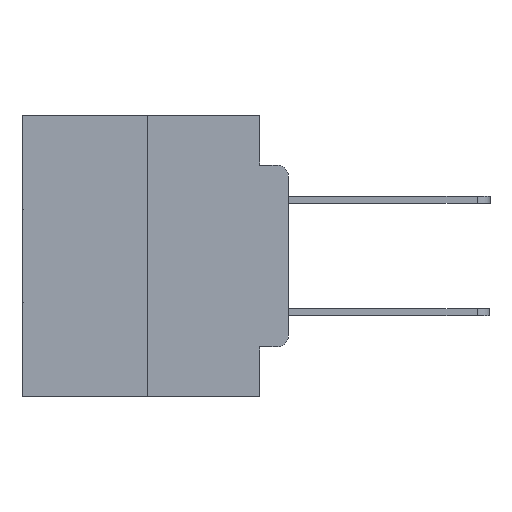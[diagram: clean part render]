
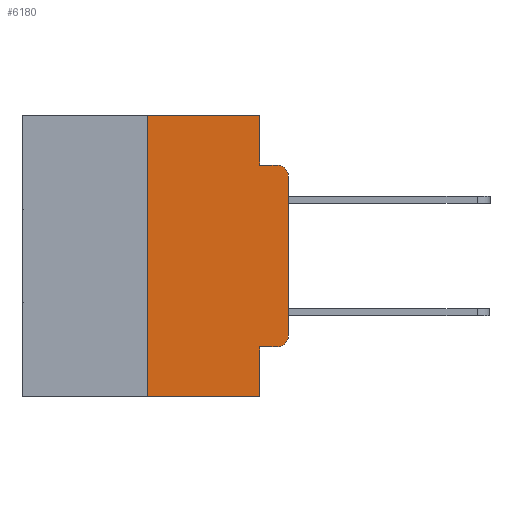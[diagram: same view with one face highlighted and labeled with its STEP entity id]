
A CAD part, left-side view. The second image highlights one B-rep face of the part: STEP entity #6180.
In plain terms, the highlighted planar face has unit normal (-1, 0, 0).
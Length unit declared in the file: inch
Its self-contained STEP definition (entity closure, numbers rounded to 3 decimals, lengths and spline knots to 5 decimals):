
#516 = ORIENTED_EDGE ( 'NONE', *, *, #24378, .F. ) ;
#706 = ORIENTED_EDGE ( 'NONE', *, *, #11833, .T. ) ;
#1183 = CARTESIAN_POINT ( 'NONE',  ( 0., 0.25, 0. ) ) ;
#1330 = ORIENTED_EDGE ( 'NONE', *, *, #25964, .T. ) ;
#2037 = CARTESIAN_POINT ( 'NONE',  ( 0., 0.02, -0.0885 ) ) ;
#2214 = EDGE_CURVE ( 'NONE', #8570, #5010, #18973, .T. ) ;
#3091 = ORIENTED_EDGE ( 'NONE', *, *, #10263, .T. ) ;
#3340 = VECTOR ( 'NONE', #28478, 39.37008 ) ;
#3778 = CARTESIAN_POINT ( 'NONE',  ( 0., 0.051, -0.5 ) ) ;
#3823 = VECTOR ( 'NONE', #24757, 39.37008 ) ;
#4241 = CARTESIAN_POINT ( 'NONE',  ( 0., 0.02, -0.1085 ) ) ;
#4290 = CARTESIAN_POINT ( 'NONE',  ( 0., 0.02, -0.3915 ) ) ;
#5010 = VERTEX_POINT ( 'NONE', #3778 ) ;
#5153 = CARTESIAN_POINT ( 'NONE',  ( 0., 0.473, -0.5 ) ) ;
#5860 = CIRCLE ( 'NONE', #20348, 0.02 ) ;
#6048 = CARTESIAN_POINT ( 'NONE',  ( 0., 0.051, 0. ) ) ;
#6180 = ADVANCED_FACE ( 'NONE', ( #27198 ), #7803, .F. ) ;
#6550 = LINE ( 'NONE', #19392, #23729 ) ;
#6603 = DIRECTION ( 'NONE',  ( 0., 0., -1. ) ) ;
#6663 = DIRECTION ( 'NONE',  ( 0., 0., -1. ) ) ;
#7413 = CIRCLE ( 'NONE', #27313, 0.02 ) ;
#7803 = PLANE ( 'NONE',  #23467 ) ;
#7943 = DIRECTION ( 'NONE',  ( 0., 0., 1. ) ) ;
#7974 = LINE ( 'NONE', #18367, #19681 ) ;
#8391 = VECTOR ( 'NONE', #12218, 39.37008 ) ;
#8570 = VERTEX_POINT ( 'NONE', #23497 ) ;
#8673 = DIRECTION ( 'NONE',  ( 0., -1., 0. ) ) ;
#9435 = ORIENTED_EDGE ( 'NONE', *, *, #27572, .T. ) ;
#9583 = LINE ( 'NONE', #26116, #3340 ) ;
#10008 = EDGE_LOOP ( 'NONE', ( #9435, #1330, #516, #18416, #14697, #24965, #27847, #11110, #706, #3091 ) ) ;
#10093 = DIRECTION ( 'NONE',  ( 0., -1., 0. ) ) ;
#10263 = EDGE_CURVE ( 'NONE', #17204, #16734, #7413, .T. ) ;
#10437 = CARTESIAN_POINT ( 'NONE',  ( 0., 0., -0.3915 ) ) ;
#10920 = CARTESIAN_POINT ( 'NONE',  ( 0., 0.051, -0.4115 ) ) ;
#11110 = ORIENTED_EDGE ( 'NONE', *, *, #14972, .F. ) ;
#11296 = VECTOR ( 'NONE', #7943, 39.37008 ) ;
#11700 = CARTESIAN_POINT ( 'NONE',  ( 0., 0., -0.1085 ) ) ;
#11833 = EDGE_CURVE ( 'NONE', #15055, #17204, #23388, .T. ) ;
#12218 = DIRECTION ( 'NONE',  ( 0., 0., -1. ) ) ;
#12506 = CARTESIAN_POINT ( 'NONE',  ( 0., 0.473, 0. ) ) ;
#14697 = ORIENTED_EDGE ( 'NONE', *, *, #24012, .F. ) ;
#14858 = DIRECTION ( 'NONE',  ( 0., 0., -1. ) ) ;
#14892 = CARTESIAN_POINT ( 'NONE',  ( 0., 0., 0. ) ) ;
#14972 = EDGE_CURVE ( 'NONE', #15055, #5010, #28731, .T. ) ;
#15055 = VERTEX_POINT ( 'NONE', #24970 ) ;
#16073 = CARTESIAN_POINT ( 'NONE',  ( 0., 0.02, -0.4115 ) ) ;
#16244 = VERTEX_POINT ( 'NONE', #18047 ) ;
#16544 = EDGE_CURVE ( 'NONE', #8570, #26471, #9583, .T. ) ;
#16734 = VERTEX_POINT ( 'NONE', #10437 ) ;
#16817 = DIRECTION ( 'NONE',  ( 0., -1., 0. ) ) ;
#17165 = VECTOR ( 'NONE', #8673, 39.37008 ) ;
#17204 = VERTEX_POINT ( 'NONE', #16073 ) ;
#17306 = VERTEX_POINT ( 'NONE', #21075 ) ;
#18047 = CARTESIAN_POINT ( 'NONE',  ( 0., 0.051, -0.0885 ) ) ;
#18113 = EDGE_CURVE ( 'NONE', #17306, #16244, #20836, .T. ) ;
#18267 = VECTOR ( 'NONE', #16817, 39.37008 ) ;
#18367 = CARTESIAN_POINT ( 'NONE',  ( 0., 0.051, -0.0885 ) ) ;
#18416 = ORIENTED_EDGE ( 'NONE', *, *, #18113, .F. ) ;
#18973 = LINE ( 'NONE', #5153, #18267 ) ;
#19392 = CARTESIAN_POINT ( 'NONE',  ( 0., 0.473, 0. ) ) ;
#19681 = VECTOR ( 'NONE', #20729, 39.37008 ) ;
#20348 = AXIS2_PLACEMENT_3D ( 'NONE', #4241, #20626, #6603 ) ;
#20626 = DIRECTION ( 'NONE',  ( -1., 0., 0. ) ) ;
#20674 = DIRECTION ( 'NONE',  ( -1., 0., 0. ) ) ;
#20729 = DIRECTION ( 'NONE',  ( 0., -1., 0. ) ) ;
#20836 = LINE ( 'NONE', #28616, #8391 ) ;
#20868 = VERTEX_POINT ( 'NONE', #2037 ) ;
#21075 = CARTESIAN_POINT ( 'NONE',  ( 0., 0.051, 0. ) ) ;
#23388 = LINE ( 'NONE', #10920, #17165 ) ;
#23467 = AXIS2_PLACEMENT_3D ( 'NONE', #12506, #28896, #14858 ) ;
#23497 = CARTESIAN_POINT ( 'NONE',  ( 0., 0.25, -0.5 ) ) ;
#23724 = LINE ( 'NONE', #14892, #11296 ) ;
#23729 = VECTOR ( 'NONE', #10093, 39.37008 ) ;
#24012 = EDGE_CURVE ( 'NONE', #26471, #17306, #6550, .T. ) ;
#24378 = EDGE_CURVE ( 'NONE', #16244, #20868, #7974, .T. ) ;
#24757 = DIRECTION ( 'NONE',  ( 0., 0., -1. ) ) ;
#24965 = ORIENTED_EDGE ( 'NONE', *, *, #16544, .F. ) ;
#24970 = CARTESIAN_POINT ( 'NONE',  ( 0., 0.051, -0.4115 ) ) ;
#25964 = EDGE_CURVE ( 'NONE', #27949, #20868, #5860, .T. ) ;
#26116 = CARTESIAN_POINT ( 'NONE',  ( 0., 0.25, 0. ) ) ;
#26471 = VERTEX_POINT ( 'NONE', #1183 ) ;
#27198 = FACE_OUTER_BOUND ( 'NONE', #10008, .T. ) ;
#27313 = AXIS2_PLACEMENT_3D ( 'NONE', #4290, #20674, #6663 ) ;
#27572 = EDGE_CURVE ( 'NONE', #16734, #27949, #23724, .T. ) ;
#27847 = ORIENTED_EDGE ( 'NONE', *, *, #2214, .T. ) ;
#27949 = VERTEX_POINT ( 'NONE', #11700 ) ;
#28478 = DIRECTION ( 'NONE',  ( 0., 0., 1. ) ) ;
#28616 = CARTESIAN_POINT ( 'NONE',  ( 0., 0.051, 0. ) ) ;
#28731 = LINE ( 'NONE', #6048, #3823 ) ;
#28896 = DIRECTION ( 'NONE',  ( 1., 0., 0. ) ) ;
